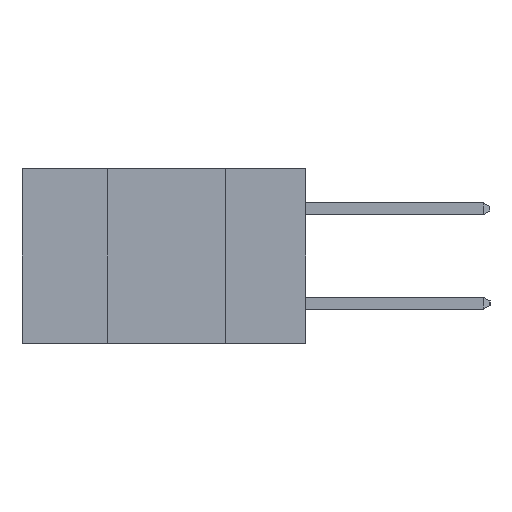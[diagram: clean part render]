
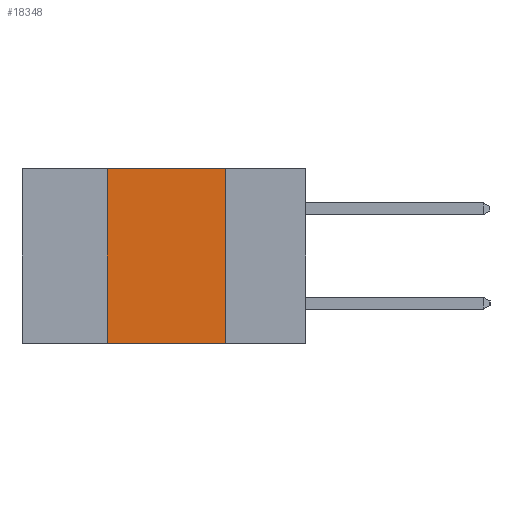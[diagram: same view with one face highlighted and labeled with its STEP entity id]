
A CAD part, left-side view. The second image highlights one B-rep face of the part: STEP entity #18348.
In plain terms, the highlighted planar face has unit normal (-1, 0, 0).
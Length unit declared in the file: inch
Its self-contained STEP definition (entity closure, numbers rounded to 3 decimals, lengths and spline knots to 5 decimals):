
#675 = LINE ( 'NONE', #15237, #14075 ) ;
#2042 = VECTOR ( 'NONE', #3875, 39.37008 ) ;
#2077 = CARTESIAN_POINT ( 'NONE',  ( 0., 0.42, -0.37 ) ) ;
#3471 = ORIENTED_EDGE ( 'NONE', *, *, #12562, .F. ) ;
#3595 = ORIENTED_EDGE ( 'NONE', *, *, #11060, .F. ) ;
#3875 = DIRECTION ( 'NONE',  ( 0., 0., 1. ) ) ;
#4077 = VECTOR ( 'NONE', #16090, 39.37008 ) ;
#4118 = EDGE_LOOP ( 'NONE', ( #6370, #3595, #3471, #22004 ) ) ;
#4255 = CARTESIAN_POINT ( 'NONE',  ( 0., 0.6, 0. ) ) ;
#5927 = FACE_OUTER_BOUND ( 'NONE', #4118, .T. ) ;
#6030 = DIRECTION ( 'NONE',  ( 0., 0., -1. ) ) ;
#6370 = ORIENTED_EDGE ( 'NONE', *, *, #6425, .F. ) ;
#6425 = EDGE_CURVE ( 'NONE', #22072, #9752, #17753, .T. ) ;
#6613 = CARTESIAN_POINT ( 'NONE',  ( 0., 0.17, -0.37 ) ) ;
#7176 = EDGE_CURVE ( 'NONE', #13133, #9752, #13813, .T. ) ;
#7555 = CARTESIAN_POINT ( 'NONE',  ( 0., 0.17, -0.37 ) ) ;
#7643 = AXIS2_PLACEMENT_3D ( 'NONE', #4255, #16273, #6030 ) ;
#8710 = CARTESIAN_POINT ( 'NONE',  ( 0., 0.42, -0.37 ) ) ;
#9752 = VERTEX_POINT ( 'NONE', #6613 ) ;
#9757 = CARTESIAN_POINT ( 'NONE',  ( 0., 0.17, 0. ) ) ;
#10214 = DIRECTION ( 'NONE',  ( 0., -1., 0. ) ) ;
#11060 = EDGE_CURVE ( 'NONE', #14864, #22072, #675, .T. ) ;
#11376 = LINE ( 'NONE', #2077, #2042 ) ;
#12246 = VECTOR ( 'NONE', #19620, 39.37008 ) ;
#12562 = EDGE_CURVE ( 'NONE', #13133, #14864, #11376, .T. ) ;
#13133 = VERTEX_POINT ( 'NONE', #8710 ) ;
#13813 = LINE ( 'NONE', #21193, #12246 ) ;
#14075 = VECTOR ( 'NONE', #10214, 39.37008 ) ;
#14864 = VERTEX_POINT ( 'NONE', #17371 ) ;
#15237 = CARTESIAN_POINT ( 'NONE',  ( 0., 0.6, 0. ) ) ;
#16090 = DIRECTION ( 'NONE',  ( 0., 0., -1. ) ) ;
#16273 = DIRECTION ( 'NONE',  ( 1., 0., 0. ) ) ;
#17371 = CARTESIAN_POINT ( 'NONE',  ( 0., 0.42, 0. ) ) ;
#17753 = LINE ( 'NONE', #7555, #4077 ) ;
#18348 = ADVANCED_FACE ( 'NONE', ( #5927 ), #21171, .F. ) ;
#19620 = DIRECTION ( 'NONE',  ( 0., -1., 0. ) ) ;
#21171 = PLANE ( 'NONE',  #7643 ) ;
#21193 = CARTESIAN_POINT ( 'NONE',  ( 0., 0.6, -0.37 ) ) ;
#22004 = ORIENTED_EDGE ( 'NONE', *, *, #7176, .T. ) ;
#22072 = VERTEX_POINT ( 'NONE', #9757 ) ;
